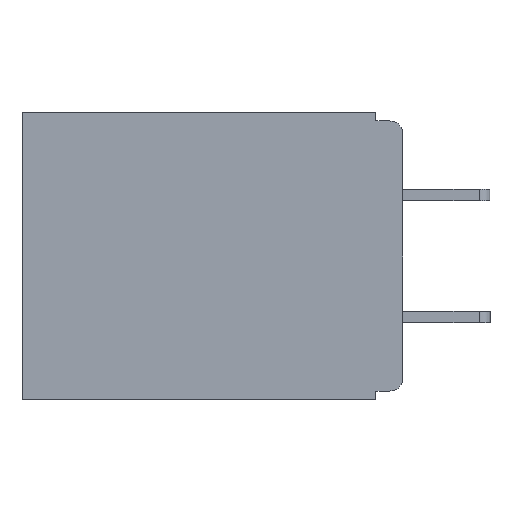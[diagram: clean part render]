
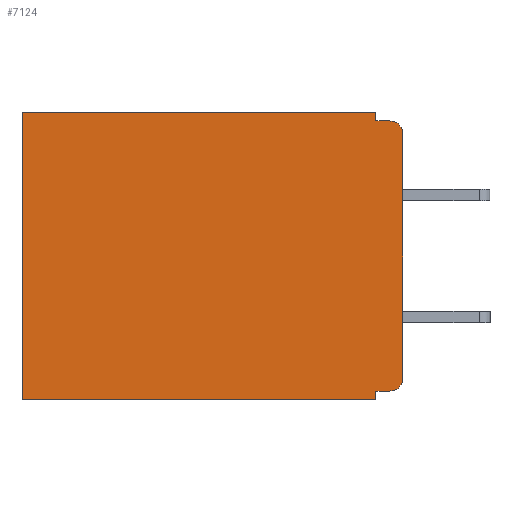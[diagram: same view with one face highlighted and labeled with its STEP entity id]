
A CAD part, left-side view. The second image highlights one B-rep face of the part: STEP entity #7124.
In plain terms, the highlighted planar face has unit normal (-1, 0, 0).
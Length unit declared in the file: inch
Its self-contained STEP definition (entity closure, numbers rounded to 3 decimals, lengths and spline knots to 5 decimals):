
#18 = DIRECTION ( 'NONE',  ( 0., 1., 0. ) ) ;
#236 = AXIS2_PLACEMENT_3D ( 'NONE', #518, #3366, #9718 ) ;
#518 = CARTESIAN_POINT ( 'NONE',  ( 0.3, 0., -0.33 ) ) ;
#559 = VERTEX_POINT ( 'NONE', #1951 ) ;
#783 = VERTEX_POINT ( 'NONE', #8987 ) ;
#991 = CARTESIAN_POINT ( 'NONE',  ( 0.3, 0.015, -0.305 ) ) ;
#1198 = CARTESIAN_POINT ( 'NONE',  ( 0.3, 0.437, 0. ) ) ;
#1286 = AXIS2_PLACEMENT_3D ( 'NONE', #8175, #2645, #9047 ) ;
#1432 = VERTEX_POINT ( 'NONE', #2019 ) ;
#1683 = VERTEX_POINT ( 'NONE', #10298 ) ;
#1706 = VERTEX_POINT ( 'NONE', #10820 ) ;
#1713 = ORIENTED_EDGE ( 'NONE', *, *, #10193, .F. ) ;
#1731 = VECTOR ( 'NONE', #10537, 39.37008 ) ;
#1735 = ORIENTED_EDGE ( 'NONE', *, *, #6855, .F. ) ;
#1951 = CARTESIAN_POINT ( 'NONE',  ( 0.3, 0.437, -0.33 ) ) ;
#1973 = LINE ( 'NONE', #8760, #9017 ) ;
#2019 = CARTESIAN_POINT ( 'NONE',  ( 0.3, 0.031, -0.33 ) ) ;
#2117 = LINE ( 'NONE', #10689, #4303 ) ;
#2311 = ORIENTED_EDGE ( 'NONE', *, *, #9136, .T. ) ;
#2347 = VECTOR ( 'NONE', #5416, 39.37008 ) ;
#2357 = ORIENTED_EDGE ( 'NONE', *, *, #7261, .F. ) ;
#2628 = EDGE_CURVE ( 'NONE', #3379, #5869, #2117, .T. ) ;
#2645 = DIRECTION ( 'NONE',  ( -1., 0., 0. ) ) ;
#2749 = ORIENTED_EDGE ( 'NONE', *, *, #10979, .F. ) ;
#2996 = CIRCLE ( 'NONE', #11566, 0.015 ) ;
#3053 = EDGE_CURVE ( 'NONE', #3066, #7397, #2996, .T. ) ;
#3066 = VERTEX_POINT ( 'NONE', #11513 ) ;
#3151 = ORIENTED_EDGE ( 'NONE', *, *, #3053, .T. ) ;
#3179 = LINE ( 'NONE', #7234, #7777 ) ;
#3366 = DIRECTION ( 'NONE',  ( 1., 0., 0. ) ) ;
#3379 = VERTEX_POINT ( 'NONE', #8063 ) ;
#3755 = CARTESIAN_POINT ( 'NONE',  ( 0.3, 0., -0.305 ) ) ;
#4024 = ORIENTED_EDGE ( 'NONE', *, *, #6736, .F. ) ;
#4154 = ORIENTED_EDGE ( 'NONE', *, *, #10640, .F. ) ;
#4303 = VECTOR ( 'NONE', #4459, 39.37008 ) ;
#4309 = DIRECTION ( 'NONE',  ( 0., 0., -1. ) ) ;
#4459 = DIRECTION ( 'NONE',  ( 0., 1., 0. ) ) ;
#4485 = DIRECTION ( 'NONE',  ( 0., 1., 0. ) ) ;
#4490 = CARTESIAN_POINT ( 'NONE',  ( 0.3, 0.031, -0.33 ) ) ;
#4540 = EDGE_LOOP ( 'NONE', ( #4154, #2311, #1735, #4024, #5231, #5708, #2357, #1713, #2749, #3151 ) ) ;
#4738 = LINE ( 'NONE', #10767, #9008 ) ;
#4887 = CARTESIAN_POINT ( 'NONE',  ( 0.3, 0.437, -0.33 ) ) ;
#5065 = LINE ( 'NONE', #4887, #7229 ) ;
#5231 = ORIENTED_EDGE ( 'NONE', *, *, #2628, .T. ) ;
#5416 = DIRECTION ( 'NONE',  ( 0., 0., -1. ) ) ;
#5441 = DIRECTION ( 'NONE',  ( 0., 0., -1. ) ) ;
#5708 = ORIENTED_EDGE ( 'NONE', *, *, #6308, .T. ) ;
#5869 = VERTEX_POINT ( 'NONE', #1198 ) ;
#6027 = CARTESIAN_POINT ( 'NONE',  ( 0.3, 0.031, -0.01 ) ) ;
#6308 = EDGE_CURVE ( 'NONE', #5869, #559, #5065, .T. ) ;
#6668 = LINE ( 'NONE', #9670, #1731 ) ;
#6736 = EDGE_CURVE ( 'NONE', #3379, #8329, #3179, .T. ) ;
#6855 = EDGE_CURVE ( 'NONE', #8329, #1706, #1973, .T. ) ;
#7124 = ADVANCED_FACE ( 'NONE', ( #8345 ), #8842, .F. ) ;
#7229 = VECTOR ( 'NONE', #4309, 39.37008 ) ;
#7234 = CARTESIAN_POINT ( 'NONE',  ( 0.3, 0.031, 0. ) ) ;
#7261 = EDGE_CURVE ( 'NONE', #1432, #559, #4738, .T. ) ;
#7397 = VERTEX_POINT ( 'NONE', #3755 ) ;
#7550 = VECTOR ( 'NONE', #18, 39.37008 ) ;
#7777 = VECTOR ( 'NONE', #11478, 39.37008 ) ;
#8063 = CARTESIAN_POINT ( 'NONE',  ( 0.3, 0.031, 0. ) ) ;
#8175 = CARTESIAN_POINT ( 'NONE',  ( 0.3, 0.015, -0.025 ) ) ;
#8329 = VERTEX_POINT ( 'NONE', #6027 ) ;
#8345 = FACE_OUTER_BOUND ( 'NONE', #4540, .T. ) ;
#8760 = CARTESIAN_POINT ( 'NONE',  ( 0.3, 0., -0.01 ) ) ;
#8842 = PLANE ( 'NONE',  #236 ) ;
#8910 = DIRECTION ( 'NONE',  ( 0., -1., 0. ) ) ;
#8987 = CARTESIAN_POINT ( 'NONE',  ( 0.3, 0.031, -0.32 ) ) ;
#9008 = VECTOR ( 'NONE', #4485, 39.37008 ) ;
#9017 = VECTOR ( 'NONE', #8910, 39.37008 ) ;
#9047 = DIRECTION ( 'NONE',  ( 0., 0., -1. ) ) ;
#9136 = EDGE_CURVE ( 'NONE', #1683, #1706, #9536, .T. ) ;
#9536 = CIRCLE ( 'NONE', #1286, 0.015 ) ;
#9647 = LINE ( 'NONE', #4490, #2347 ) ;
#9670 = CARTESIAN_POINT ( 'NONE',  ( 0.3, 0., -0.33 ) ) ;
#9718 = DIRECTION ( 'NONE',  ( 0., 0., -1. ) ) ;
#9906 = LINE ( 'NONE', #10942, #7550 ) ;
#10193 = EDGE_CURVE ( 'NONE', #783, #1432, #9647, .T. ) ;
#10298 = CARTESIAN_POINT ( 'NONE',  ( 0.3, 0., -0.025 ) ) ;
#10537 = DIRECTION ( 'NONE',  ( 0., 0., -1. ) ) ;
#10640 = EDGE_CURVE ( 'NONE', #1683, #7397, #6668, .T. ) ;
#10689 = CARTESIAN_POINT ( 'NONE',  ( 0.3, 0., 0. ) ) ;
#10767 = CARTESIAN_POINT ( 'NONE',  ( 0.3, 0., -0.33 ) ) ;
#10820 = CARTESIAN_POINT ( 'NONE',  ( 0.3, 0.015, -0.01 ) ) ;
#10870 = DIRECTION ( 'NONE',  ( -1., 0., 0. ) ) ;
#10942 = CARTESIAN_POINT ( 'NONE',  ( 0.3, 0., -0.32 ) ) ;
#10979 = EDGE_CURVE ( 'NONE', #3066, #783, #9906, .T. ) ;
#11478 = DIRECTION ( 'NONE',  ( 0., 0., -1. ) ) ;
#11513 = CARTESIAN_POINT ( 'NONE',  ( 0.3, 0.015, -0.32 ) ) ;
#11566 = AXIS2_PLACEMENT_3D ( 'NONE', #991, #10870, #5441 ) ;
